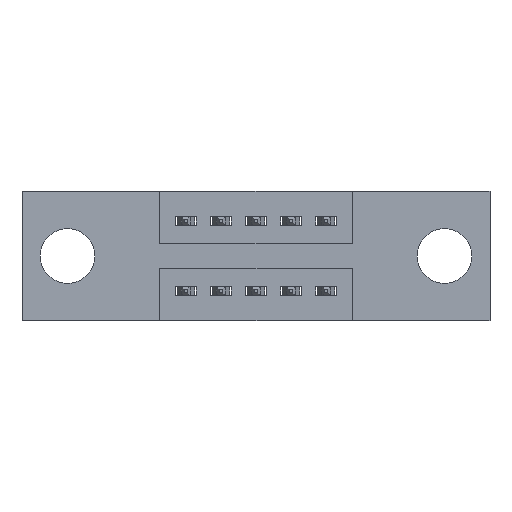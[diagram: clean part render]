
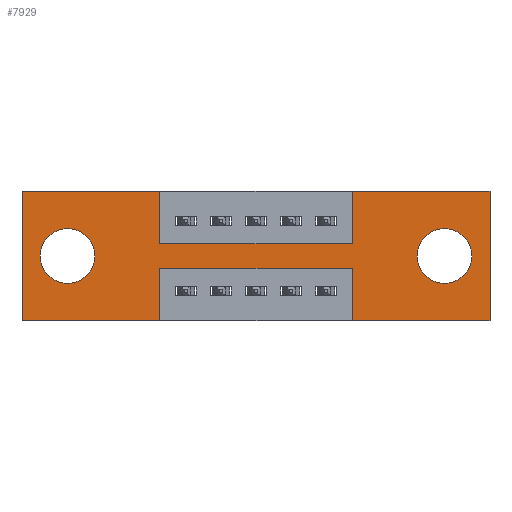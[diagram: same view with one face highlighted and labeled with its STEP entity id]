
A CAD part, front view. The second image highlights one B-rep face of the part: STEP entity #7929.
In plain terms, the highlighted planar face has unit normal (0, -1, 0).
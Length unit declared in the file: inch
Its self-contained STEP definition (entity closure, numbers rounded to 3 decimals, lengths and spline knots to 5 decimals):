
#13 = CARTESIAN_POINT ( 'NONE',  ( 1.205, 0., -0.107 ) ) ;
#42 = EDGE_CURVE ( 'NONE', #948, #4875, #1444, .T. ) ;
#44 = DIRECTION ( 'NONE',  ( -1., 0., 0. ) ) ;
#374 = CIRCLE ( 'NONE', #5563, 0.078 ) ;
#540 = CIRCLE ( 'NONE', #7376, 0.078 ) ;
#569 = EDGE_CURVE ( 'NONE', #3677, #4735, #4707, .T. ) ;
#641 = LINE ( 'NONE', #5275, #3664 ) ;
#843 = FACE_BOUND ( 'NONE', #4583, .T. ) ;
#936 = ORIENTED_EDGE ( 'NONE', *, *, #7903, .F. ) ;
#948 = VERTEX_POINT ( 'NONE', #8281 ) ;
#1032 = DIRECTION ( 'NONE',  ( 0., 1., 0. ) ) ;
#1093 = EDGE_LOOP ( 'NONE', ( #3877, #2219, #8171, #4147, #936, #4210, #1448, #8643, #5042, #5975, #8113, #4486 ) ) ;
#1111 = CARTESIAN_POINT ( 'NONE',  ( 0.9425, 0., -0.37 ) ) ;
#1231 = DIRECTION ( 'NONE',  ( 0., 0., -1. ) ) ;
#1278 = DIRECTION ( 'NONE',  ( 0., 0., 1. ) ) ;
#1444 = LINE ( 'NONE', #1111, #4378 ) ;
#1448 = ORIENTED_EDGE ( 'NONE', *, *, #8447, .F. ) ;
#1452 = DIRECTION ( 'NONE',  ( 0., 0., 1. ) ) ;
#1453 = CARTESIAN_POINT ( 'NONE',  ( 0., 0., 0. ) ) ;
#1489 = ORIENTED_EDGE ( 'NONE', *, *, #5624, .T. ) ;
#1498 = VECTOR ( 'NONE', #3422, 39.37008 ) ;
#1629 = DIRECTION ( 'NONE',  ( 0., 0., -1. ) ) ;
#1660 = CARTESIAN_POINT ( 'NONE',  ( 0.3925, 0., -0.22 ) ) ;
#1694 = DIRECTION ( 'NONE',  ( -1., 0., 0. ) ) ;
#1696 = DIRECTION ( 'NONE',  ( 0., 0., 1. ) ) ;
#1725 = DIRECTION ( 'NONE',  ( 1., 0., 0. ) ) ;
#1768 = LINE ( 'NONE', #8605, #4812 ) ;
#1809 = EDGE_CURVE ( 'NONE', #4534, #2598, #5716, .T. ) ;
#1864 = EDGE_CURVE ( 'NONE', #8003, #2143, #6255, .T. ) ;
#2051 = EDGE_CURVE ( 'NONE', #6669, #3677, #8311, .T. ) ;
#2143 = VERTEX_POINT ( 'NONE', #2429 ) ;
#2219 = ORIENTED_EDGE ( 'NONE', *, *, #6370, .F. ) ;
#2305 = CARTESIAN_POINT ( 'NONE',  ( 0., 0., 0. ) ) ;
#2367 = DIRECTION ( 'NONE',  ( 1., 0., 0. ) ) ;
#2429 = CARTESIAN_POINT ( 'NONE',  ( 0.13, 0., -0.263 ) ) ;
#2454 = CARTESIAN_POINT ( 'NONE',  ( 0.3925, 0., -0.22 ) ) ;
#2598 = VERTEX_POINT ( 'NONE', #3104 ) ;
#2681 = FACE_BOUND ( 'NONE', #8788, .T. ) ;
#2899 = CARTESIAN_POINT ( 'NONE',  ( 0.9425, 0., 0. ) ) ;
#3036 = DIRECTION ( 'NONE',  ( -1., 0., 0. ) ) ;
#3043 = ORIENTED_EDGE ( 'NONE', *, *, #7308, .T. ) ;
#3055 = DIRECTION ( 'NONE',  ( 0., 0., -1. ) ) ;
#3104 = CARTESIAN_POINT ( 'NONE',  ( 0.3925, 0., -0.37 ) ) ;
#3145 = ORIENTED_EDGE ( 'NONE', *, *, #1864, .T. ) ;
#3148 = CARTESIAN_POINT ( 'NONE',  ( 0.13, 0., -0.107 ) ) ;
#3182 = CARTESIAN_POINT ( 'NONE',  ( 0., 0., 0. ) ) ;
#3260 = EDGE_CURVE ( 'NONE', #7506, #5499, #6021, .T. ) ;
#3286 = EDGE_CURVE ( 'NONE', #4735, #4553, #641, .T. ) ;
#3422 = DIRECTION ( 'NONE',  ( 1., 0., 0. ) ) ;
#3442 = LINE ( 'NONE', #2899, #6893 ) ;
#3471 = DIRECTION ( 'NONE',  ( 0., 0., -1. ) ) ;
#3518 = CARTESIAN_POINT ( 'NONE',  ( 0.9425, 0., -0.22 ) ) ;
#3527 = CARTESIAN_POINT ( 'NONE',  ( 0.13, 0., -0.185 ) ) ;
#3664 = VECTOR ( 'NONE', #1231, 39.37008 ) ;
#3677 = VERTEX_POINT ( 'NONE', #1453 ) ;
#3749 = PLANE ( 'NONE',  #5636 ) ;
#3762 = CARTESIAN_POINT ( 'NONE',  ( 0.13, 0., -0.185 ) ) ;
#3830 = CARTESIAN_POINT ( 'NONE',  ( 1.205, 0., -0.185 ) ) ;
#3877 = ORIENTED_EDGE ( 'NONE', *, *, #1809, .F. ) ;
#4022 = VECTOR ( 'NONE', #5768, 39.37008 ) ;
#4147 = ORIENTED_EDGE ( 'NONE', *, *, #7150, .F. ) ;
#4188 = DIRECTION ( 'NONE',  ( 0., 0., 1. ) ) ;
#4197 = CARTESIAN_POINT ( 'NONE',  ( 0., 0., -0.37 ) ) ;
#4210 = ORIENTED_EDGE ( 'NONE', *, *, #3260, .F. ) ;
#4213 = CARTESIAN_POINT ( 'NONE',  ( 0.3925, 0., -0.37 ) ) ;
#4378 = VECTOR ( 'NONE', #1278, 39.37008 ) ;
#4462 = CARTESIAN_POINT ( 'NONE',  ( 0.9425, 0., -0.15 ) ) ;
#4486 = ORIENTED_EDGE ( 'NONE', *, *, #6381, .F. ) ;
#4534 = VERTEX_POINT ( 'NONE', #2454 ) ;
#4553 = VERTEX_POINT ( 'NONE', #7859 ) ;
#4573 = VECTOR ( 'NONE', #5899, 39.37008 ) ;
#4583 = EDGE_LOOP ( 'NONE', ( #3145, #3043 ) ) ;
#4707 = LINE ( 'NONE', #2305, #4916 ) ;
#4735 = VERTEX_POINT ( 'NONE', #4923 ) ;
#4772 = LINE ( 'NONE', #5102, #4022 ) ;
#4790 = VECTOR ( 'NONE', #3471, 39.37008 ) ;
#4812 = VECTOR ( 'NONE', #1694, 39.37008 ) ;
#4875 = VERTEX_POINT ( 'NONE', #3518 ) ;
#4885 = ORIENTED_EDGE ( 'NONE', *, *, #5410, .T. ) ;
#4916 = VECTOR ( 'NONE', #2367, 39.37008 ) ;
#4923 = CARTESIAN_POINT ( 'NONE',  ( 0.3925, 0., 0. ) ) ;
#5042 = ORIENTED_EDGE ( 'NONE', *, *, #3286, .F. ) ;
#5102 = CARTESIAN_POINT ( 'NONE',  ( 1.335, 0., 0. ) ) ;
#5130 = CARTESIAN_POINT ( 'NONE',  ( 0., 0., 0. ) ) ;
#5275 = CARTESIAN_POINT ( 'NONE',  ( 0.3925, 0., 0. ) ) ;
#5410 = EDGE_CURVE ( 'NONE', #7311, #6725, #7924, .T. ) ;
#5465 = AXIS2_PLACEMENT_3D ( 'NONE', #3527, #8342, #4188 ) ;
#5499 = VERTEX_POINT ( 'NONE', #5691 ) ;
#5563 = AXIS2_PLACEMENT_3D ( 'NONE', #3830, #6599, #8637 ) ;
#5624 = EDGE_CURVE ( 'NONE', #6725, #7311, #374, .T. ) ;
#5636 = AXIS2_PLACEMENT_3D ( 'NONE', #7252, #7898, #3055 ) ;
#5691 = CARTESIAN_POINT ( 'NONE',  ( 1.335, 0., 0. ) ) ;
#5716 = LINE ( 'NONE', #4213, #4790 ) ;
#5751 = DIRECTION ( 'NONE',  ( 0., 1., 0. ) ) ;
#5768 = DIRECTION ( 'NONE',  ( 0., 0., -1. ) ) ;
#5847 = VERTEX_POINT ( 'NONE', #6838 ) ;
#5899 = DIRECTION ( 'NONE',  ( 0., 0., 1. ) ) ;
#5975 = ORIENTED_EDGE ( 'NONE', *, *, #569, .F. ) ;
#6021 = LINE ( 'NONE', #3182, #6888 ) ;
#6236 = CARTESIAN_POINT ( 'NONE',  ( 0.3925, 0., -0.15 ) ) ;
#6255 = CIRCLE ( 'NONE', #5465, 0.078 ) ;
#6370 = EDGE_CURVE ( 'NONE', #4875, #4534, #8893, .T. ) ;
#6381 = EDGE_CURVE ( 'NONE', #2598, #6669, #1768, .T. ) ;
#6437 = CARTESIAN_POINT ( 'NONE',  ( 1.205, 0., -0.263 ) ) ;
#6474 = CARTESIAN_POINT ( 'NONE',  ( 1.205, 0., -0.185 ) ) ;
#6574 = LINE ( 'NONE', #6236, #1498 ) ;
#6599 = DIRECTION ( 'NONE',  ( 0., 1., 0. ) ) ;
#6669 = VERTEX_POINT ( 'NONE', #7406 ) ;
#6725 = VERTEX_POINT ( 'NONE', #13 ) ;
#6838 = CARTESIAN_POINT ( 'NONE',  ( 1.335, 0., -0.37 ) ) ;
#6888 = VECTOR ( 'NONE', #1725, 39.37008 ) ;
#6893 = VECTOR ( 'NONE', #1452, 39.37008 ) ;
#6896 = LINE ( 'NONE', #4197, #7552 ) ;
#7010 = EDGE_CURVE ( 'NONE', #4553, #7325, #6574, .T. ) ;
#7150 = EDGE_CURVE ( 'NONE', #5847, #948, #6896, .T. ) ;
#7252 = CARTESIAN_POINT ( 'NONE',  ( 0., 0., -0.37 ) ) ;
#7308 = EDGE_CURVE ( 'NONE', #2143, #8003, #540, .T. ) ;
#7311 = VERTEX_POINT ( 'NONE', #6437 ) ;
#7325 = VERTEX_POINT ( 'NONE', #4462 ) ;
#7376 = AXIS2_PLACEMENT_3D ( 'NONE', #3762, #1032, #1696 ) ;
#7406 = CARTESIAN_POINT ( 'NONE',  ( 0., 0., -0.37 ) ) ;
#7506 = VERTEX_POINT ( 'NONE', #8673 ) ;
#7552 = VECTOR ( 'NONE', #44, 39.37008 ) ;
#7638 = AXIS2_PLACEMENT_3D ( 'NONE', #6474, #5751, #1629 ) ;
#7652 = FACE_OUTER_BOUND ( 'NONE', #1093, .T. ) ;
#7859 = CARTESIAN_POINT ( 'NONE',  ( 0.3925, 0., -0.15 ) ) ;
#7898 = DIRECTION ( 'NONE',  ( 0., -1., 0. ) ) ;
#7903 = EDGE_CURVE ( 'NONE', #5499, #5847, #4772, .T. ) ;
#7924 = CIRCLE ( 'NONE', #7638, 0.078 ) ;
#7929 = ADVANCED_FACE ( 'NONE', ( #2681, #843, #7652 ), #3749, .T. ) ;
#8003 = VERTEX_POINT ( 'NONE', #3148 ) ;
#8113 = ORIENTED_EDGE ( 'NONE', *, *, #2051, .F. ) ;
#8171 = ORIENTED_EDGE ( 'NONE', *, *, #42, .F. ) ;
#8281 = CARTESIAN_POINT ( 'NONE',  ( 0.9425, 0., -0.37 ) ) ;
#8311 = LINE ( 'NONE', #5130, #4573 ) ;
#8342 = DIRECTION ( 'NONE',  ( 0., 1., 0. ) ) ;
#8446 = VECTOR ( 'NONE', #3036, 39.37008 ) ;
#8447 = EDGE_CURVE ( 'NONE', #7325, #7506, #3442, .T. ) ;
#8605 = CARTESIAN_POINT ( 'NONE',  ( 0., 0., -0.37 ) ) ;
#8637 = DIRECTION ( 'NONE',  ( 0., 0., -1. ) ) ;
#8643 = ORIENTED_EDGE ( 'NONE', *, *, #7010, .F. ) ;
#8673 = CARTESIAN_POINT ( 'NONE',  ( 0.9425, 0., 0. ) ) ;
#8788 = EDGE_LOOP ( 'NONE', ( #1489, #4885 ) ) ;
#8893 = LINE ( 'NONE', #1660, #8446 ) ;
